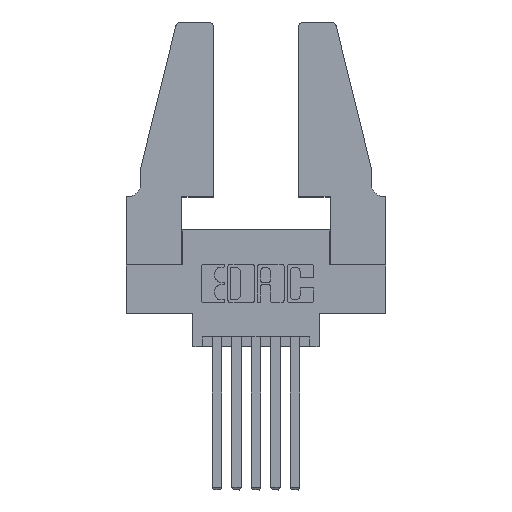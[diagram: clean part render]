
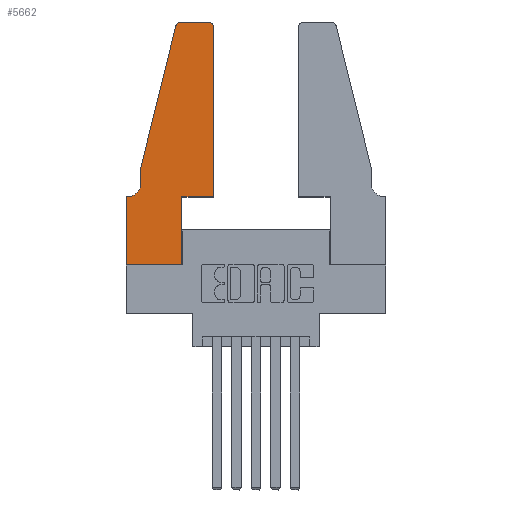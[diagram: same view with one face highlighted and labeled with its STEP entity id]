
A CAD part, top view. The second image highlights one B-rep face of the part: STEP entity #5662.
In plain terms, the highlighted planar face has unit normal (0, 0, 1).
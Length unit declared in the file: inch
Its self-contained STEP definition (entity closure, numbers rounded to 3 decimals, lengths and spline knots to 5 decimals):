
#36 = CARTESIAN_POINT ( 'NONE',  ( 0.0755, 0.5, 0.37 ) ) ;
#92 = CARTESIAN_POINT ( 'NONE',  ( 0.0755, 0.42, 0.37 ) ) ;
#241 = VERTEX_POINT ( 'NONE', #689 ) ;
#505 = VERTEX_POINT ( 'NONE', #92 ) ;
#515 = CARTESIAN_POINT ( 'NONE',  ( 0.284, 1.22, 0.37 ) ) ;
#588 = CARTESIAN_POINT ( 'NONE',  ( 0.4505, 0.35, 0.37 ) ) ;
#617 = EDGE_LOOP ( 'NONE', ( #2236, #7805, #2040, #914, #2819, #852, #5692, #3621, #10438, #9633, #7209, #2627 ) ) ;
#689 = CARTESIAN_POINT ( 'NONE',  ( 0.25487, 1.22718, 0.37 ) ) ;
#852 = ORIENTED_EDGE ( 'NONE', *, *, #8254, .T. ) ;
#856 = CARTESIAN_POINT ( 'NONE',  ( 0., 0.35, 0.37 ) ) ;
#912 = VECTOR ( 'NONE', #2691, 39.37008 ) ;
#914 = ORIENTED_EDGE ( 'NONE', *, *, #7879, .T. ) ;
#979 = DIRECTION ( 'NONE',  ( 1., 0., 0. ) ) ;
#990 = VECTOR ( 'NONE', #2295, 39.37008 ) ;
#1120 = AXIS2_PLACEMENT_3D ( 'NONE', #8343, #3309, #9169 ) ;
#1158 = VERTEX_POINT ( 'NONE', #6943 ) ;
#1215 = VECTOR ( 'NONE', #4360, 39.37008 ) ;
#1313 = CARTESIAN_POINT ( 'NONE',  ( 0.0055, 0.35, 0.37 ) ) ;
#1477 = LINE ( 'NONE', #8677, #9658 ) ;
#1488 = DIRECTION ( 'NONE',  ( 1., 0., 0. ) ) ;
#1520 = LINE ( 'NONE', #6893, #912 ) ;
#1554 = DIRECTION ( 'NONE',  ( 1., 0., 0. ) ) ;
#1788 = CARTESIAN_POINT ( 'NONE',  ( 0.2865, 0.35, 0.37 ) ) ;
#2040 = ORIENTED_EDGE ( 'NONE', *, *, #3894, .T. ) ;
#2236 = ORIENTED_EDGE ( 'NONE', *, *, #9288, .T. ) ;
#2295 = DIRECTION ( 'NONE',  ( -1., 0., 0. ) ) ;
#2322 = DIRECTION ( 'NONE',  ( 0., -1., 0. ) ) ;
#2455 = DIRECTION ( 'NONE',  ( 0., 0., 1. ) ) ;
#2473 = PLANE ( 'NONE',  #1120 ) ;
#2477 = VERTEX_POINT ( 'NONE', #1788 ) ;
#2627 = ORIENTED_EDGE ( 'NONE', *, *, #6921, .T. ) ;
#2691 = DIRECTION ( 'NONE',  ( -0.239, -0.971, 0. ) ) ;
#2741 = VERTEX_POINT ( 'NONE', #856 ) ;
#2819 = ORIENTED_EDGE ( 'NONE', *, *, #4529, .T. ) ;
#3008 = AXIS2_PLACEMENT_3D ( 'NONE', #7499, #2455, #8326 ) ;
#3010 = VERTEX_POINT ( 'NONE', #8425 ) ;
#3098 = LINE ( 'NONE', #8159, #990 ) ;
#3164 = CARTESIAN_POINT ( 'NONE',  ( 0., 0., 0.37 ) ) ;
#3180 = VERTEX_POINT ( 'NONE', #9512 ) ;
#3305 = CARTESIAN_POINT ( 'NONE',  ( 0.0755, 0.35, 0.37 ) ) ;
#3309 = DIRECTION ( 'NONE',  ( 0., 0., 1. ) ) ;
#3444 = CIRCLE ( 'NONE', #4927, 0.07 ) ;
#3495 = CARTESIAN_POINT ( 'NONE',  ( 0.4505, 0.35, 0.37 ) ) ;
#3533 = VERTEX_POINT ( 'NONE', #1313 ) ;
#3545 = CARTESIAN_POINT ( 'NONE',  ( 0.0055, 0.42, 0.37 ) ) ;
#3621 = ORIENTED_EDGE ( 'NONE', *, *, #10800, .T. ) ;
#3877 = EDGE_CURVE ( 'NONE', #4993, #3180, #8010, .T. ) ;
#3894 = EDGE_CURVE ( 'NONE', #241, #3010, #1520, .T. ) ;
#4223 = VECTOR ( 'NONE', #1554, 39.37008 ) ;
#4360 = DIRECTION ( 'NONE',  ( 0., 1., 0. ) ) ;
#4427 = DIRECTION ( 'NONE',  ( -1., 0., 0. ) ) ;
#4529 = EDGE_CURVE ( 'NONE', #505, #3533, #3444, .T. ) ;
#4609 = CIRCLE ( 'NONE', #3008, 0.03 ) ;
#4637 = VECTOR ( 'NONE', #2322, 39.37008 ) ;
#4927 = AXIS2_PLACEMENT_3D ( 'NONE', #3545, #9406, #4427 ) ;
#4982 = CARTESIAN_POINT ( 'NONE',  ( 0.4505, 0.35, 0.37 ) ) ;
#4993 = VERTEX_POINT ( 'NONE', #4982 ) ;
#5011 = CARTESIAN_POINT ( 'NONE',  ( 0., 0., 0.37 ) ) ;
#5536 = EDGE_CURVE ( 'NONE', #2741, #10563, #6862, .T. ) ;
#5592 = EDGE_CURVE ( 'NONE', #10173, #241, #8545, .T. ) ;
#5662 = ADVANCED_FACE ( 'NONE', ( #8009 ), #2473, .T. ) ;
#5692 = ORIENTED_EDGE ( 'NONE', *, *, #5536, .T. ) ;
#5797 = VECTOR ( 'NONE', #7233, 39.37008 ) ;
#6171 = LINE ( 'NONE', #36, #6440 ) ;
#6232 = EDGE_CURVE ( 'NONE', #2477, #4993, #6460, .T. ) ;
#6440 = VECTOR ( 'NONE', #7036, 39.37008 ) ;
#6460 = LINE ( 'NONE', #588, #4223 ) ;
#6569 = EDGE_CURVE ( 'NONE', #1158, #2477, #10206, .T. ) ;
#6602 = DIRECTION ( 'NONE',  ( 0., 0., 1. ) ) ;
#6691 = LINE ( 'NONE', #3305, #7197 ) ;
#6862 = LINE ( 'NONE', #3164, #4637 ) ;
#6893 = CARTESIAN_POINT ( 'NONE',  ( 0.0755, 0.5, 0.37 ) ) ;
#6921 = EDGE_CURVE ( 'NONE', #3180, #9614, #4609, .T. ) ;
#6943 = CARTESIAN_POINT ( 'NONE',  ( 0.2865, 0., 0.37 ) ) ;
#6988 = CARTESIAN_POINT ( 'NONE',  ( 0.4205, 1.25, 0.37 ) ) ;
#7036 = DIRECTION ( 'NONE',  ( 0., -1., 0. ) ) ;
#7197 = VECTOR ( 'NONE', #8339, 39.37008 ) ;
#7209 = ORIENTED_EDGE ( 'NONE', *, *, #3877, .T. ) ;
#7233 = DIRECTION ( 'NONE',  ( 0., 1., 0. ) ) ;
#7499 = CARTESIAN_POINT ( 'NONE',  ( 0.4205, 1.22, 0.37 ) ) ;
#7805 = ORIENTED_EDGE ( 'NONE', *, *, #5592, .T. ) ;
#7879 = EDGE_CURVE ( 'NONE', #3010, #505, #6171, .T. ) ;
#8009 = FACE_OUTER_BOUND ( 'NONE', #617, .T. ) ;
#8010 = LINE ( 'NONE', #3495, #1215 ) ;
#8159 = CARTESIAN_POINT ( 'NONE',  ( 0.2605, 1.25, 0.37 ) ) ;
#8189 = AXIS2_PLACEMENT_3D ( 'NONE', #515, #6602, #1488 ) ;
#8254 = EDGE_CURVE ( 'NONE', #3533, #2741, #6691, .T. ) ;
#8326 = DIRECTION ( 'NONE',  ( 1., 0., 0. ) ) ;
#8339 = DIRECTION ( 'NONE',  ( -1., 0., 0. ) ) ;
#8343 = CARTESIAN_POINT ( 'NONE',  ( 0., 0.35, 0.37 ) ) ;
#8425 = CARTESIAN_POINT ( 'NONE',  ( 0.0755, 0.5, 0.37 ) ) ;
#8545 = CIRCLE ( 'NONE', #8189, 0.03 ) ;
#8677 = CARTESIAN_POINT ( 'NONE',  ( 0., 0., 0.37 ) ) ;
#9169 = DIRECTION ( 'NONE',  ( 1., 0., 0. ) ) ;
#9288 = EDGE_CURVE ( 'NONE', #9614, #10173, #3098, .T. ) ;
#9406 = DIRECTION ( 'NONE',  ( 0., 0., -1. ) ) ;
#9468 = CARTESIAN_POINT ( 'NONE',  ( 0.284, 1.25, 0.37 ) ) ;
#9512 = CARTESIAN_POINT ( 'NONE',  ( 0.4505, 1.22, 0.37 ) ) ;
#9614 = VERTEX_POINT ( 'NONE', #6988 ) ;
#9633 = ORIENTED_EDGE ( 'NONE', *, *, #6232, .T. ) ;
#9658 = VECTOR ( 'NONE', #979, 39.37008 ) ;
#9691 = CARTESIAN_POINT ( 'NONE',  ( 0.2865, 0.35, 0.37 ) ) ;
#10173 = VERTEX_POINT ( 'NONE', #9468 ) ;
#10206 = LINE ( 'NONE', #9691, #5797 ) ;
#10438 = ORIENTED_EDGE ( 'NONE', *, *, #6569, .T. ) ;
#10563 = VERTEX_POINT ( 'NONE', #5011 ) ;
#10800 = EDGE_CURVE ( 'NONE', #10563, #1158, #1477, .T. ) ;
